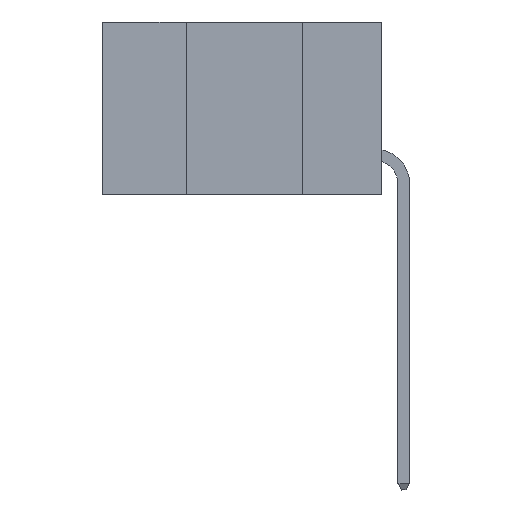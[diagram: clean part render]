
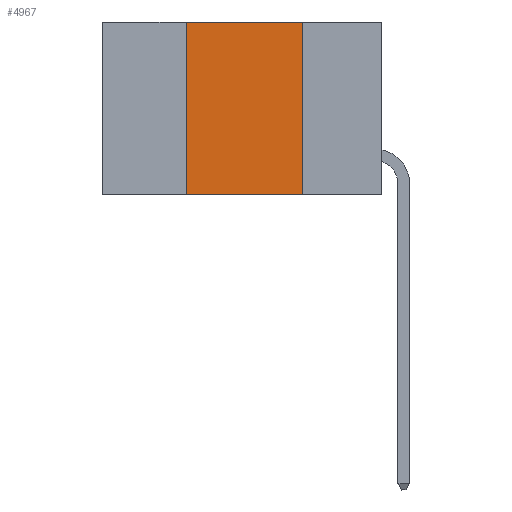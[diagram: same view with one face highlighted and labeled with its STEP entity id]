
A CAD part, left-side view. The second image highlights one B-rep face of the part: STEP entity #4967.
In plain terms, the highlighted planar face has unit normal (-1, 0, 0).
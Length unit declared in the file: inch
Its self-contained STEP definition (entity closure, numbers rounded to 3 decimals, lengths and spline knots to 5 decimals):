
#654 = LINE ( 'NONE', #14104, #16646 ) ;
#1070 = VECTOR ( 'NONE', #19170, 39.37008 ) ;
#3135 = ORIENTED_EDGE ( 'NONE', *, *, #29077, .T. ) ;
#3363 = CARTESIAN_POINT ( 'NONE',  ( 0., 0.42, 0. ) ) ;
#3736 = DIRECTION ( 'NONE',  ( 0., 0., -1. ) ) ;
#4128 = AXIS2_PLACEMENT_3D ( 'NONE', #17286, #17189, #3736 ) ;
#4967 = ADVANCED_FACE ( 'NONE', ( #5574 ), #10660, .F. ) ;
#5574 = FACE_OUTER_BOUND ( 'NONE', #7044, .T. ) ;
#7044 = EDGE_LOOP ( 'NONE', ( #10003, #23264, #10191, #3135 ) ) ;
#7088 = DIRECTION ( 'NONE',  ( 0., 0., -1. ) ) ;
#7151 = LINE ( 'NONE', #3363, #1070 ) ;
#10003 = ORIENTED_EDGE ( 'NONE', *, *, #25915, .F. ) ;
#10191 = ORIENTED_EDGE ( 'NONE', *, *, #16365, .F. ) ;
#10660 = PLANE ( 'NONE',  #4128 ) ;
#11229 = VERTEX_POINT ( 'NONE', #19684 ) ;
#12868 = CARTESIAN_POINT ( 'NONE',  ( 0., 0.6, -0.37 ) ) ;
#13168 = LINE ( 'NONE', #24847, #23376 ) ;
#13960 = CARTESIAN_POINT ( 'NONE',  ( 0., 0.42, -0.37 ) ) ;
#14104 = CARTESIAN_POINT ( 'NONE',  ( 0., 0.6, 0. ) ) ;
#14909 = VERTEX_POINT ( 'NONE', #13960 ) ;
#16365 = EDGE_CURVE ( 'NONE', #14909, #11229, #7151, .T. ) ;
#16646 = VECTOR ( 'NONE', #18646, 39.37008 ) ;
#17189 = DIRECTION ( 'NONE',  ( 1., 0., 0. ) ) ;
#17286 = CARTESIAN_POINT ( 'NONE',  ( 0., 0.6, 0. ) ) ;
#18052 = VERTEX_POINT ( 'NONE', #20774 ) ;
#18646 = DIRECTION ( 'NONE',  ( 0., -1., 0. ) ) ;
#19170 = DIRECTION ( 'NONE',  ( 0., 0., 1. ) ) ;
#19684 = CARTESIAN_POINT ( 'NONE',  ( 0., 0.42, 0. ) ) ;
#20774 = CARTESIAN_POINT ( 'NONE',  ( 0., 0.17, -0.37 ) ) ;
#22818 = EDGE_CURVE ( 'NONE', #11229, #29055, #654, .T. ) ;
#23264 = ORIENTED_EDGE ( 'NONE', *, *, #22818, .F. ) ;
#23376 = VECTOR ( 'NONE', #7088, 39.37008 ) ;
#23805 = DIRECTION ( 'NONE',  ( 0., -1., 0. ) ) ;
#24847 = CARTESIAN_POINT ( 'NONE',  ( 0., 0.17, 0. ) ) ;
#25915 = EDGE_CURVE ( 'NONE', #29055, #18052, #13168, .T. ) ;
#26743 = LINE ( 'NONE', #12868, #27098 ) ;
#27098 = VECTOR ( 'NONE', #23805, 39.37008 ) ;
#28493 = CARTESIAN_POINT ( 'NONE',  ( 0., 0.17, 0. ) ) ;
#29055 = VERTEX_POINT ( 'NONE', #28493 ) ;
#29077 = EDGE_CURVE ( 'NONE', #14909, #18052, #26743, .T. ) ;
